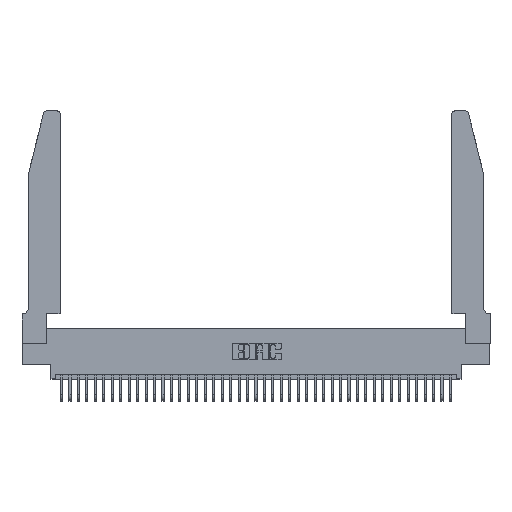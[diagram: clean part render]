
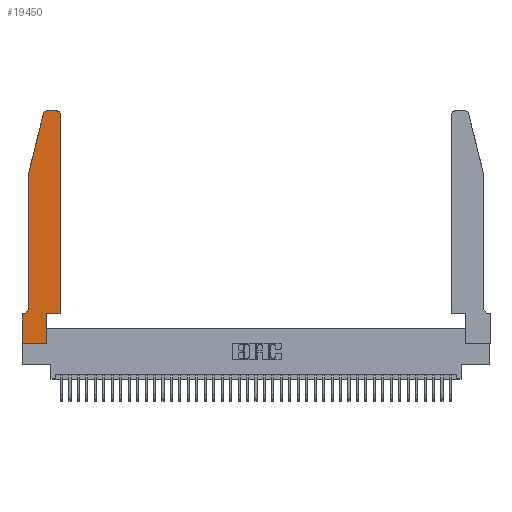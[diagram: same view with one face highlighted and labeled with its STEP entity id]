
A CAD part, top view. The second image highlights one B-rep face of the part: STEP entity #19450.
In plain terms, the highlighted planar face has unit normal (0, 0, 1).
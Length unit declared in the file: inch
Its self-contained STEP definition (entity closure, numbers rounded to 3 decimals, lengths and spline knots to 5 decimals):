
#197 = CARTESIAN_POINT ( 'NONE',  ( 0.4205, 2.75, 0.37 ) ) ;
#1220 = EDGE_CURVE ( 'NONE', #17704, #21406, #11322, .T. ) ;
#1894 = DIRECTION ( 'NONE',  ( 0., 0., 1. ) ) ;
#2381 = ORIENTED_EDGE ( 'NONE', *, *, #10447, .T. ) ;
#2422 = EDGE_CURVE ( 'NONE', #18854, #13047, #24070, .T. ) ;
#2754 = VECTOR ( 'NONE', #6978, 39.37008 ) ;
#2904 = VERTEX_POINT ( 'NONE', #32915 ) ;
#2978 = DIRECTION ( 'NONE',  ( 0., 0., 1. ) ) ;
#3459 = LINE ( 'NONE', #38242, #35008 ) ;
#4425 = EDGE_CURVE ( 'NONE', #20531, #7156, #9674, .T. ) ;
#4891 = CIRCLE ( 'NONE', #19073, 0.07 ) ;
#5170 = ORIENTED_EDGE ( 'NONE', *, *, #24243, .T. ) ;
#5358 = DIRECTION ( 'NONE',  ( 0., 0., -1. ) ) ;
#5436 = LINE ( 'NONE', #12301, #36987 ) ;
#6288 = CARTESIAN_POINT ( 'NONE',  ( 0.25487, 2.72718, 0.37 ) ) ;
#6978 = DIRECTION ( 'NONE',  ( -1., 0., 0. ) ) ;
#7156 = VERTEX_POINT ( 'NONE', #14006 ) ;
#7242 = EDGE_CURVE ( 'NONE', #36313, #27681, #4891, .T. ) ;
#7787 = VECTOR ( 'NONE', #30053, 39.37008 ) ;
#7795 = CARTESIAN_POINT ( 'NONE',  ( 0.4505, 0.35, 0.37 ) ) ;
#8396 = ORIENTED_EDGE ( 'NONE', *, *, #4425, .T. ) ;
#9491 = CARTESIAN_POINT ( 'NONE',  ( 0.0755, 0.35, 0.37 ) ) ;
#9674 = LINE ( 'NONE', #33045, #7787 ) ;
#10447 = EDGE_CURVE ( 'NONE', #25606, #20531, #20305, .T. ) ;
#10735 = DIRECTION ( 'NONE',  ( 0., 0., 1. ) ) ;
#10831 = DIRECTION ( 'NONE',  ( 0., -1., 0. ) ) ;
#10886 = LINE ( 'NONE', #34365, #2754 ) ;
#10908 = CARTESIAN_POINT ( 'NONE',  ( 0.4505, 2.72, 0.37 ) ) ;
#11013 = ORIENTED_EDGE ( 'NONE', *, *, #12005, .T. ) ;
#11046 = ORIENTED_EDGE ( 'NONE', *, *, #22960, .T. ) ;
#11322 = LINE ( 'NONE', #31273, #26584 ) ;
#11899 = LINE ( 'NONE', #24464, #19005 ) ;
#12005 = EDGE_CURVE ( 'NONE', #37766, #36877, #18524, .T. ) ;
#12227 = VECTOR ( 'NONE', #26333, 39.37008 ) ;
#12301 = CARTESIAN_POINT ( 'NONE',  ( 0.4505, 0.35, 0.37 ) ) ;
#12334 = DIRECTION ( 'NONE',  ( -0.239, -0.971, 0. ) ) ;
#12572 = AXIS2_PLACEMENT_3D ( 'NONE', #29026, #10735, #32134 ) ;
#12646 = EDGE_CURVE ( 'NONE', #13047, #37766, #10886, .T. ) ;
#13047 = VERTEX_POINT ( 'NONE', #197 ) ;
#13564 = CARTESIAN_POINT ( 'NONE',  ( 0.2865, 0.35, 0.37 ) ) ;
#14006 = CARTESIAN_POINT ( 'NONE',  ( 0.2865, 0., 0.37 ) ) ;
#14032 = CARTESIAN_POINT ( 'NONE',  ( 0., 0.35, 0.37 ) ) ;
#14039 = CARTESIAN_POINT ( 'NONE',  ( 0., 0., 0.37 ) ) ;
#16314 = EDGE_CURVE ( 'NONE', #2904, #36313, #3459, .T. ) ;
#16632 = DIRECTION ( 'NONE',  ( 0., 1., 0. ) ) ;
#17704 = VERTEX_POINT ( 'NONE', #38549 ) ;
#17832 = LINE ( 'NONE', #13564, #31256 ) ;
#18500 = ORIENTED_EDGE ( 'NONE', *, *, #12646, .T. ) ;
#18524 = CIRCLE ( 'NONE', #12572, 0.03 ) ;
#18829 = LINE ( 'NONE', #9491, #26999 ) ;
#18854 = VERTEX_POINT ( 'NONE', #10908 ) ;
#19005 = VECTOR ( 'NONE', #12334, 39.37008 ) ;
#19073 = AXIS2_PLACEMENT_3D ( 'NONE', #23599, #5358, #26696 ) ;
#19444 = FACE_OUTER_BOUND ( 'NONE', #26240, .T. ) ;
#19450 = ADVANCED_FACE ( 'NONE', ( #19444 ), #20125, .T. ) ;
#19647 = CARTESIAN_POINT ( 'NONE',  ( 0., 0., 0.37 ) ) ;
#20125 = PLANE ( 'NONE',  #37228 ) ;
#20156 = ORIENTED_EDGE ( 'NONE', *, *, #1220, .T. ) ;
#20269 = CARTESIAN_POINT ( 'NONE',  ( 0., 0.35, 0.37 ) ) ;
#20305 = LINE ( 'NONE', #14039, #12227 ) ;
#20362 = ORIENTED_EDGE ( 'NONE', *, *, #7242, .T. ) ;
#20531 = VERTEX_POINT ( 'NONE', #19647 ) ;
#21245 = CARTESIAN_POINT ( 'NONE',  ( 0.4205, 2.72, 0.37 ) ) ;
#21406 = VERTEX_POINT ( 'NONE', #7795 ) ;
#21601 = ORIENTED_EDGE ( 'NONE', *, *, #2422, .T. ) ;
#21963 = EDGE_CURVE ( 'NONE', #7156, #17704, #17832, .T. ) ;
#22859 = CARTESIAN_POINT ( 'NONE',  ( 0.284, 2.75, 0.37 ) ) ;
#22960 = EDGE_CURVE ( 'NONE', #21406, #18854, #5436, .T. ) ;
#23227 = DIRECTION ( 'NONE',  ( 1., 0., 0. ) ) ;
#23599 = CARTESIAN_POINT ( 'NONE',  ( 0.0055, 0.42, 0.37 ) ) ;
#24070 = CIRCLE ( 'NONE', #32650, 0.03 ) ;
#24243 = EDGE_CURVE ( 'NONE', #27681, #25606, #18829, .T. ) ;
#24318 = DIRECTION ( 'NONE',  ( 1., 0., 0. ) ) ;
#24464 = CARTESIAN_POINT ( 'NONE',  ( 0.0755, 2., 0.37 ) ) ;
#25606 = VERTEX_POINT ( 'NONE', #20269 ) ;
#25618 = CARTESIAN_POINT ( 'NONE',  ( 0.0055, 0.35, 0.37 ) ) ;
#26240 = EDGE_LOOP ( 'NONE', ( #18500, #11013, #33445, #33211, #20362, #5170, #2381, #8396, #28461, #20156, #11046, #21601 ) ) ;
#26333 = DIRECTION ( 'NONE',  ( 0., -1., 0. ) ) ;
#26584 = VECTOR ( 'NONE', #27598, 39.37008 ) ;
#26696 = DIRECTION ( 'NONE',  ( -1., 0., 0. ) ) ;
#26999 = VECTOR ( 'NONE', #33954, 39.37008 ) ;
#27598 = DIRECTION ( 'NONE',  ( 1., 0., 0. ) ) ;
#27681 = VERTEX_POINT ( 'NONE', #25618 ) ;
#28461 = ORIENTED_EDGE ( 'NONE', *, *, #21963, .T. ) ;
#29026 = CARTESIAN_POINT ( 'NONE',  ( 0.284, 2.72, 0.37 ) ) ;
#30053 = DIRECTION ( 'NONE',  ( 1., 0., 0. ) ) ;
#30736 = DIRECTION ( 'NONE',  ( 0., 1., 0. ) ) ;
#31256 = VECTOR ( 'NONE', #16632, 39.37008 ) ;
#31273 = CARTESIAN_POINT ( 'NONE',  ( 0.4505, 0.35, 0.37 ) ) ;
#32134 = DIRECTION ( 'NONE',  ( 1., 0., 0. ) ) ;
#32650 = AXIS2_PLACEMENT_3D ( 'NONE', #21245, #2978, #24318 ) ;
#32915 = CARTESIAN_POINT ( 'NONE',  ( 0.0755, 2., 0.37 ) ) ;
#33045 = CARTESIAN_POINT ( 'NONE',  ( 0., 0., 0.37 ) ) ;
#33211 = ORIENTED_EDGE ( 'NONE', *, *, #16314, .T. ) ;
#33445 = ORIENTED_EDGE ( 'NONE', *, *, #36140, .T. ) ;
#33954 = DIRECTION ( 'NONE',  ( -1., 0., 0. ) ) ;
#34365 = CARTESIAN_POINT ( 'NONE',  ( 0.2605, 2.75, 0.37 ) ) ;
#35008 = VECTOR ( 'NONE', #10831, 39.37008 ) ;
#36140 = EDGE_CURVE ( 'NONE', #36877, #2904, #11899, .T. ) ;
#36313 = VERTEX_POINT ( 'NONE', #37611 ) ;
#36877 = VERTEX_POINT ( 'NONE', #6288 ) ;
#36987 = VECTOR ( 'NONE', #30736, 39.37008 ) ;
#37228 = AXIS2_PLACEMENT_3D ( 'NONE', #14032, #1894, #23227 ) ;
#37611 = CARTESIAN_POINT ( 'NONE',  ( 0.0755, 0.42, 0.37 ) ) ;
#37766 = VERTEX_POINT ( 'NONE', #22859 ) ;
#38242 = CARTESIAN_POINT ( 'NONE',  ( 0.0755, 2., 0.37 ) ) ;
#38549 = CARTESIAN_POINT ( 'NONE',  ( 0.2865, 0.35, 0.37 ) ) ;
